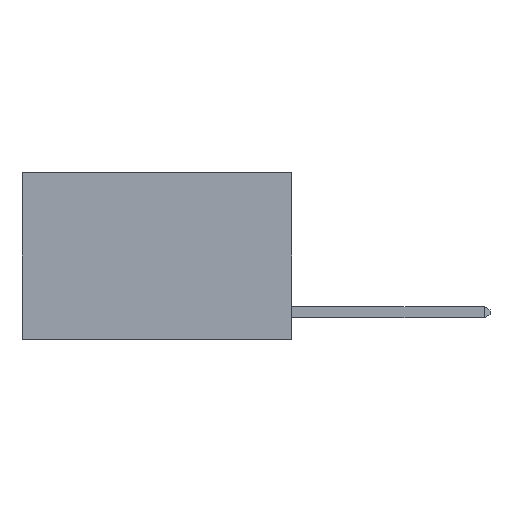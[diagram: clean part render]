
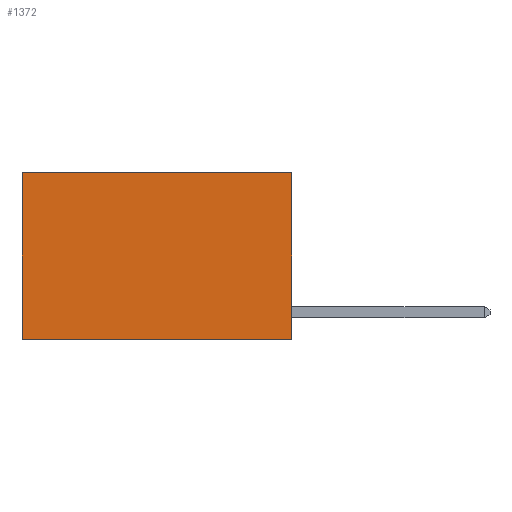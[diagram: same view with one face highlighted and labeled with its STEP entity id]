
A CAD part, left-side view. The second image highlights one B-rep face of the part: STEP entity #1372.
In plain terms, the highlighted planar face has unit normal (-1, 0, 0).
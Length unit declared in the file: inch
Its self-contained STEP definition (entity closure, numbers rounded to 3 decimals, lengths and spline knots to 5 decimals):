
#44 = VERTEX_POINT ( 'NONE', #707 ) ;
#338 = CARTESIAN_POINT ( 'NONE',  ( 0.2625, 0., 0. ) ) ;
#707 = CARTESIAN_POINT ( 'NONE',  ( 0.2625, 0., -0.37 ) ) ;
#1363 = CARTESIAN_POINT ( 'NONE',  ( 0.2625, 0.6, 0. ) ) ;
#1372 = ADVANCED_FACE ( 'NONE', ( #6180 ), #4339, .F. ) ;
#1504 = EDGE_CURVE ( 'NONE', #44, #8242, #7374, .T. ) ;
#1549 = VERTEX_POINT ( 'NONE', #7304 ) ;
#1844 = CARTESIAN_POINT ( 'NONE',  ( 0.2625, 0., 0. ) ) ;
#1882 = CARTESIAN_POINT ( 'NONE',  ( 0.2625, 0., -0.37 ) ) ;
#2544 = ORIENTED_EDGE ( 'NONE', *, *, #7219, .T. ) ;
#2817 = VECTOR ( 'NONE', #7745, 39.37008 ) ;
#2863 = ORIENTED_EDGE ( 'NONE', *, *, #1504, .F. ) ;
#3473 = CARTESIAN_POINT ( 'NONE',  ( 0.2625, 0.6, -0.37 ) ) ;
#3874 = VERTEX_POINT ( 'NONE', #6919 ) ;
#3940 = AXIS2_PLACEMENT_3D ( 'NONE', #10484, #10879, #7531 ) ;
#4339 = PLANE ( 'NONE',  #3940 ) ;
#5365 = EDGE_LOOP ( 'NONE', ( #2544, #2863, #6355, #7957 ) ) ;
#5595 = EDGE_CURVE ( 'NONE', #3874, #1549, #7241, .T. ) ;
#6180 = FACE_OUTER_BOUND ( 'NONE', #5365, .T. ) ;
#6355 = ORIENTED_EDGE ( 'NONE', *, *, #11233, .F. ) ;
#6919 = CARTESIAN_POINT ( 'NONE',  ( 0.2625, 0., 0. ) ) ;
#7021 = DIRECTION ( 'NONE',  ( 0., 1., 0. ) ) ;
#7219 = EDGE_CURVE ( 'NONE', #1549, #8242, #7337, .T. ) ;
#7241 = LINE ( 'NONE', #1844, #9297 ) ;
#7304 = CARTESIAN_POINT ( 'NONE',  ( 0.2625, 0.6, 0. ) ) ;
#7337 = LINE ( 'NONE', #1363, #11165 ) ;
#7374 = LINE ( 'NONE', #1882, #2817 ) ;
#7531 = DIRECTION ( 'NONE',  ( 0., 0., -1. ) ) ;
#7745 = DIRECTION ( 'NONE',  ( 0., 1., 0. ) ) ;
#7957 = ORIENTED_EDGE ( 'NONE', *, *, #5595, .T. ) ;
#8076 = VECTOR ( 'NONE', #9918, 39.37008 ) ;
#8242 = VERTEX_POINT ( 'NONE', #3473 ) ;
#9297 = VECTOR ( 'NONE', #7021, 39.37008 ) ;
#9918 = DIRECTION ( 'NONE',  ( 0., 0., -1. ) ) ;
#10006 = DIRECTION ( 'NONE',  ( 0., 0., -1. ) ) ;
#10403 = LINE ( 'NONE', #338, #8076 ) ;
#10484 = CARTESIAN_POINT ( 'NONE',  ( 0.2625, 0., 0. ) ) ;
#10879 = DIRECTION ( 'NONE',  ( 1., 0., 0. ) ) ;
#11165 = VECTOR ( 'NONE', #10006, 39.37008 ) ;
#11233 = EDGE_CURVE ( 'NONE', #3874, #44, #10403, .T. ) ;
